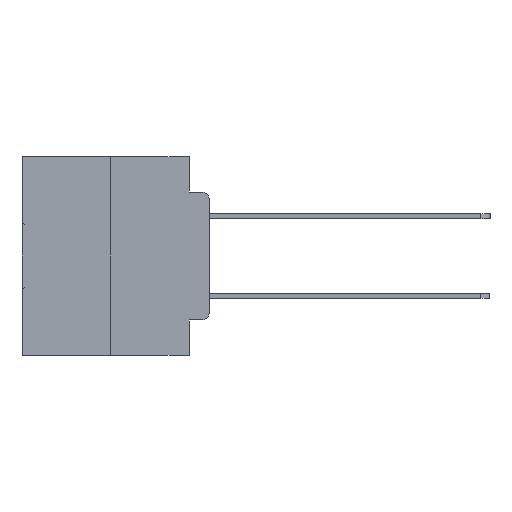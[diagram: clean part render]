
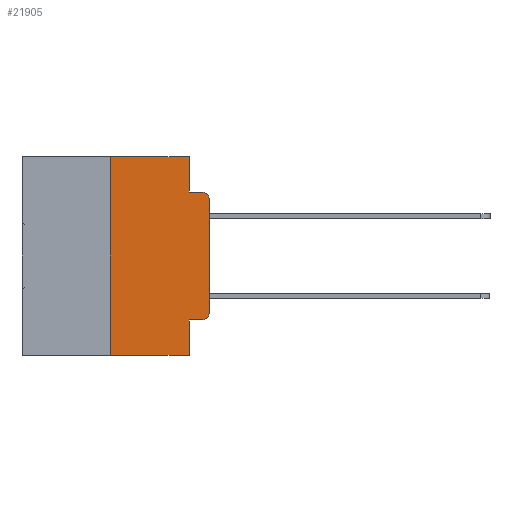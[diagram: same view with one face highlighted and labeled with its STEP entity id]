
A CAD part, left-side view. The second image highlights one B-rep face of the part: STEP entity #21905.
In plain terms, the highlighted planar face has unit normal (-1, 0, 0).
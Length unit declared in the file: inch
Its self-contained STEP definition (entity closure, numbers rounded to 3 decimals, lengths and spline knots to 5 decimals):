
#282 = VECTOR ( 'NONE', #9857, 39.37008 ) ;
#420 = VERTEX_POINT ( 'NONE', #24847 ) ;
#461 = EDGE_CURVE ( 'NONE', #7840, #420, #28574, .T. ) ;
#734 = VECTOR ( 'NONE', #5379, 39.37008 ) ;
#755 = VECTOR ( 'NONE', #12038, 39.37008 ) ;
#1589 = ORIENTED_EDGE ( 'NONE', *, *, #7071, .T. ) ;
#1596 = EDGE_CURVE ( 'NONE', #22024, #32627, #14959, .T. ) ;
#1644 = CARTESIAN_POINT ( 'NONE',  ( 0., 0.473, 0. ) ) ;
#1965 = DIRECTION ( 'NONE',  ( 0., -1., 0. ) ) ;
#1980 = VERTEX_POINT ( 'NONE', #26968 ) ;
#2217 = CARTESIAN_POINT ( 'NONE',  ( 0., 0.25, 0. ) ) ;
#2524 = DIRECTION ( 'NONE',  ( 0., 0., -1. ) ) ;
#2898 = ORIENTED_EDGE ( 'NONE', *, *, #31965, .T. ) ;
#3316 = DIRECTION ( 'NONE',  ( -1., 0., 0. ) ) ;
#3643 = VECTOR ( 'NONE', #1965, 39.37008 ) ;
#3907 = VERTEX_POINT ( 'NONE', #27283 ) ;
#4014 = ORIENTED_EDGE ( 'NONE', *, *, #34183, .T. ) ;
#5379 = DIRECTION ( 'NONE',  ( 0., -1., 0. ) ) ;
#6268 = CARTESIAN_POINT ( 'NONE',  ( 0., 0.02, -0.0885 ) ) ;
#6479 = LINE ( 'NONE', #7596, #11983 ) ;
#6658 = DIRECTION ( 'NONE',  ( 0., 0., -1. ) ) ;
#6761 = CARTESIAN_POINT ( 'NONE',  ( 0., 0.051, 0. ) ) ;
#6798 = FACE_OUTER_BOUND ( 'NONE', #20439, .T. ) ;
#7071 = EDGE_CURVE ( 'NONE', #20434, #22024, #6479, .T. ) ;
#7596 = CARTESIAN_POINT ( 'NONE',  ( 0., 0., 0. ) ) ;
#7735 = EDGE_CURVE ( 'NONE', #1980, #24444, #11487, .T. ) ;
#7840 = VERTEX_POINT ( 'NONE', #19787 ) ;
#9857 = DIRECTION ( 'NONE',  ( 0., -1., 0. ) ) ;
#10879 = LINE ( 'NONE', #30947, #3643 ) ;
#11487 = LINE ( 'NONE', #2217, #32380 ) ;
#11671 = ORIENTED_EDGE ( 'NONE', *, *, #13809, .T. ) ;
#11983 = VECTOR ( 'NONE', #26149, 39.37008 ) ;
#12038 = DIRECTION ( 'NONE',  ( 0., 0., -1. ) ) ;
#12369 = CARTESIAN_POINT ( 'NONE',  ( 0., 0.25, 0. ) ) ;
#12951 = ORIENTED_EDGE ( 'NONE', *, *, #7735, .F. ) ;
#13809 = EDGE_CURVE ( 'NONE', #7840, #3907, #10879, .T. ) ;
#14391 = ORIENTED_EDGE ( 'NONE', *, *, #18037, .F. ) ;
#14842 = CIRCLE ( 'NONE', #17892, 0.02 ) ;
#14959 = CIRCLE ( 'NONE', #15243, 0.02 ) ;
#15243 = AXIS2_PLACEMENT_3D ( 'NONE', #28368, #28438, #26982 ) ;
#16263 = VECTOR ( 'NONE', #6658, 39.37008 ) ;
#16663 = EDGE_CURVE ( 'NONE', #31527, #23063, #27437, .T. ) ;
#17048 = ORIENTED_EDGE ( 'NONE', *, *, #1596, .T. ) ;
#17892 = AXIS2_PLACEMENT_3D ( 'NONE', #19349, #3316, #22027 ) ;
#18037 = EDGE_CURVE ( 'NONE', #24444, #31527, #21633, .T. ) ;
#18249 = LINE ( 'NONE', #21593, #32145 ) ;
#18562 = DIRECTION ( 'NONE',  ( 1., 0., 0. ) ) ;
#19349 = CARTESIAN_POINT ( 'NONE',  ( 0., 0.02, -0.3915 ) ) ;
#19787 = CARTESIAN_POINT ( 'NONE',  ( 0., 0.051, -0.4115 ) ) ;
#20429 = LINE ( 'NONE', #21344, #734 ) ;
#20434 = VERTEX_POINT ( 'NONE', #28306 ) ;
#20439 = EDGE_LOOP ( 'NONE', ( #1589, #17048, #21329, #25957, #14391, #12951, #4014, #22528, #11671, #2898 ) ) ;
#21329 = ORIENTED_EDGE ( 'NONE', *, *, #28963, .F. ) ;
#21344 = CARTESIAN_POINT ( 'NONE',  ( 0., 0.051, -0.0885 ) ) ;
#21593 = CARTESIAN_POINT ( 'NONE',  ( 0., 0.473, -0.5 ) ) ;
#21633 = LINE ( 'NONE', #1644, #282 ) ;
#21905 = ADVANCED_FACE ( 'NONE', ( #6798 ), #26425, .F. ) ;
#22024 = VERTEX_POINT ( 'NONE', #26981 ) ;
#22027 = DIRECTION ( 'NONE',  ( 0., 0., -1. ) ) ;
#22528 = ORIENTED_EDGE ( 'NONE', *, *, #461, .F. ) ;
#23063 = VERTEX_POINT ( 'NONE', #27642 ) ;
#23599 = DIRECTION ( 'NONE',  ( 0., 0., 1. ) ) ;
#23803 = CARTESIAN_POINT ( 'NONE',  ( 0., 0.473, 0. ) ) ;
#24265 = DIRECTION ( 'NONE',  ( 0., -1., 0. ) ) ;
#24444 = VERTEX_POINT ( 'NONE', #12369 ) ;
#24847 = CARTESIAN_POINT ( 'NONE',  ( 0., 0.051, -0.5 ) ) ;
#24923 = CARTESIAN_POINT ( 'NONE',  ( 0., 0.051, 0. ) ) ;
#25957 = ORIENTED_EDGE ( 'NONE', *, *, #16663, .F. ) ;
#26149 = DIRECTION ( 'NONE',  ( 0., 0., 1. ) ) ;
#26425 = PLANE ( 'NONE',  #32423 ) ;
#26968 = CARTESIAN_POINT ( 'NONE',  ( 0., 0.25, -0.5 ) ) ;
#26981 = CARTESIAN_POINT ( 'NONE',  ( 0., 0., -0.1085 ) ) ;
#26982 = DIRECTION ( 'NONE',  ( 0., 0., -1. ) ) ;
#27283 = CARTESIAN_POINT ( 'NONE',  ( 0., 0.02, -0.4115 ) ) ;
#27437 = LINE ( 'NONE', #27784, #755 ) ;
#27642 = CARTESIAN_POINT ( 'NONE',  ( 0., 0.051, -0.0885 ) ) ;
#27784 = CARTESIAN_POINT ( 'NONE',  ( 0., 0.051, 0. ) ) ;
#28306 = CARTESIAN_POINT ( 'NONE',  ( 0., 0., -0.3915 ) ) ;
#28368 = CARTESIAN_POINT ( 'NONE',  ( 0., 0.02, -0.1085 ) ) ;
#28438 = DIRECTION ( 'NONE',  ( -1., 0., 0. ) ) ;
#28574 = LINE ( 'NONE', #6761, #16263 ) ;
#28963 = EDGE_CURVE ( 'NONE', #23063, #32627, #20429, .T. ) ;
#30947 = CARTESIAN_POINT ( 'NONE',  ( 0., 0.051, -0.4115 ) ) ;
#31527 = VERTEX_POINT ( 'NONE', #24923 ) ;
#31965 = EDGE_CURVE ( 'NONE', #3907, #20434, #14842, .T. ) ;
#32145 = VECTOR ( 'NONE', #24265, 39.37008 ) ;
#32380 = VECTOR ( 'NONE', #23599, 39.37008 ) ;
#32423 = AXIS2_PLACEMENT_3D ( 'NONE', #23803, #18562, #2524 ) ;
#32627 = VERTEX_POINT ( 'NONE', #6268 ) ;
#34183 = EDGE_CURVE ( 'NONE', #1980, #420, #18249, .T. ) ;
